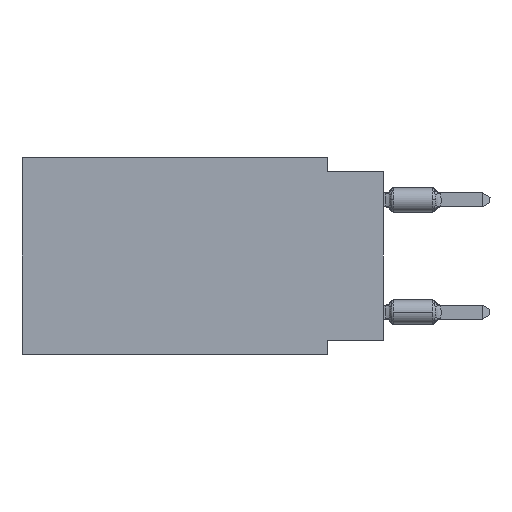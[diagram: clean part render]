
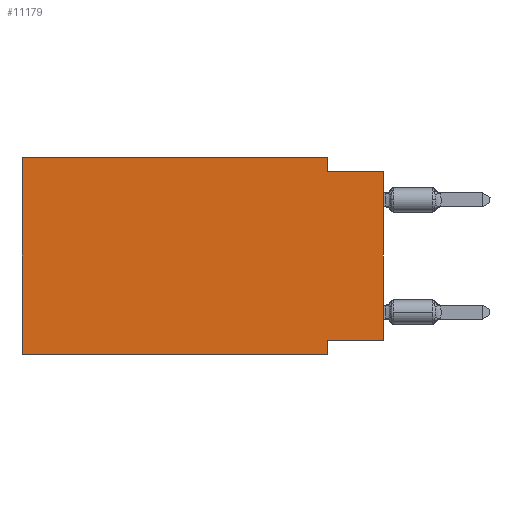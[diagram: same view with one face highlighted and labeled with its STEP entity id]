
A CAD part, left-side view. The second image highlights one B-rep face of the part: STEP entity #11179.
In plain terms, the highlighted planar face has unit normal (-1, 0, 0).
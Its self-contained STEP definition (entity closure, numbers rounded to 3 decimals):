
#908 = DIRECTION ( 'NONE',  ( 0., 0., -1. ) ) ;
#1858 = LINE ( 'NONE', #10172, #21087 ) ;
#2636 = DIRECTION ( 'NONE',  ( 0., 1., 0. ) ) ;
#2695 = VERTEX_POINT ( 'NONE', #25205 ) ;
#3220 = LINE ( 'NONE', #24862, #30269 ) ;
#4189 = VECTOR ( 'NONE', #20116, 1000. ) ;
#4745 = VERTEX_POINT ( 'NONE', #19446 ) ;
#5129 = LINE ( 'NONE', #21970, #16484 ) ;
#6118 = CARTESIAN_POINT ( 'NONE',  ( 0., 0., -0.635 ) ) ;
#7174 = DIRECTION ( 'NONE',  ( 0., 0., -1. ) ) ;
#7586 = ORIENTED_EDGE ( 'NONE', *, *, #32528, .F. ) ;
#7727 = CARTESIAN_POINT ( 'NONE',  ( 0., 2.54, -8.255 ) ) ;
#9203 = EDGE_CURVE ( 'NONE', #30146, #4745, #13804, .T. ) ;
#9887 = DIRECTION ( 'NONE',  ( 0., 0., -1. ) ) ;
#10009 = DIRECTION ( 'NONE',  ( 0., -1., 0. ) ) ;
#10089 = CARTESIAN_POINT ( 'NONE',  ( 0., 0., -8.255 ) ) ;
#10172 = CARTESIAN_POINT ( 'NONE',  ( 0., 16.383, 0. ) ) ;
#10361 = CARTESIAN_POINT ( 'NONE',  ( 0., 16.383, -8.89 ) ) ;
#11179 = ADVANCED_FACE ( 'NONE', ( #23169 ), #29033, .F. ) ;
#12017 = ORIENTED_EDGE ( 'NONE', *, *, #25292, .F. ) ;
#12849 = CARTESIAN_POINT ( 'NONE',  ( 0., 16.383, 0. ) ) ;
#13617 = ORIENTED_EDGE ( 'NONE', *, *, #9203, .T. ) ;
#13804 = LINE ( 'NONE', #29809, #14140 ) ;
#14010 = EDGE_CURVE ( 'NONE', #21302, #32073, #32221, .T. ) ;
#14140 = VECTOR ( 'NONE', #21966, 1000. ) ;
#16460 = VERTEX_POINT ( 'NONE', #17766 ) ;
#16484 = VECTOR ( 'NONE', #2636, 1000. ) ;
#16853 = EDGE_CURVE ( 'NONE', #17032, #32073, #20550, .T. ) ;
#16901 = CARTESIAN_POINT ( 'NONE',  ( 0., 16.383, 0. ) ) ;
#17032 = VERTEX_POINT ( 'NONE', #7727 ) ;
#17487 = LINE ( 'NONE', #6118, #27730 ) ;
#17766 = CARTESIAN_POINT ( 'NONE',  ( 0., 2.54, 0. ) ) ;
#19446 = CARTESIAN_POINT ( 'NONE',  ( 0., 0., -0.635 ) ) ;
#19974 = ORIENTED_EDGE ( 'NONE', *, *, #16853, .F. ) ;
#20116 = DIRECTION ( 'NONE',  ( 0., -1., 0. ) ) ;
#20370 = CARTESIAN_POINT ( 'NONE',  ( 0., 2.54, -8.89 ) ) ;
#20550 = LINE ( 'NONE', #31224, #26715 ) ;
#21087 = VECTOR ( 'NONE', #28681, 1000. ) ;
#21229 = ORIENTED_EDGE ( 'NONE', *, *, #22100, .F. ) ;
#21302 = VERTEX_POINT ( 'NONE', #29407 ) ;
#21428 = ORIENTED_EDGE ( 'NONE', *, *, #29186, .F. ) ;
#21966 = DIRECTION ( 'NONE',  ( 0., 0., 1. ) ) ;
#21970 = CARTESIAN_POINT ( 'NONE',  ( 0., 0., -8.255 ) ) ;
#22100 = EDGE_CURVE ( 'NONE', #30146, #17032, #5129, .T. ) ;
#23169 = FACE_OUTER_BOUND ( 'NONE', #23328, .T. ) ;
#23328 = EDGE_LOOP ( 'NONE', ( #13617, #7586, #12017, #30321, #21428, #34111, #19974, #21229 ) ) ;
#24862 = CARTESIAN_POINT ( 'NONE',  ( 0., 2.54, 0. ) ) ;
#24988 = EDGE_CURVE ( 'NONE', #31687, #16460, #34009, .T. ) ;
#25205 = CARTESIAN_POINT ( 'NONE',  ( 0., 2.54, -0.635 ) ) ;
#25292 = EDGE_CURVE ( 'NONE', #16460, #2695, #3220, .T. ) ;
#25366 = VECTOR ( 'NONE', #10009, 1000. ) ;
#26715 = VECTOR ( 'NONE', #9887, 1000. ) ;
#27730 = VECTOR ( 'NONE', #27982, 1000. ) ;
#27982 = DIRECTION ( 'NONE',  ( 0., -1., 0. ) ) ;
#28133 = AXIS2_PLACEMENT_3D ( 'NONE', #12849, #28684, #7174 ) ;
#28655 = CARTESIAN_POINT ( 'NONE',  ( 0., 16.383, 0. ) ) ;
#28681 = DIRECTION ( 'NONE',  ( 0., 0., 1. ) ) ;
#28684 = DIRECTION ( 'NONE',  ( 1., 0., 0. ) ) ;
#29033 = PLANE ( 'NONE',  #28133 ) ;
#29186 = EDGE_CURVE ( 'NONE', #21302, #31687, #1858, .T. ) ;
#29407 = CARTESIAN_POINT ( 'NONE',  ( 0., 16.383, -8.89 ) ) ;
#29809 = CARTESIAN_POINT ( 'NONE',  ( 0., 0., 0. ) ) ;
#30146 = VERTEX_POINT ( 'NONE', #10089 ) ;
#30269 = VECTOR ( 'NONE', #908, 1000. ) ;
#30321 = ORIENTED_EDGE ( 'NONE', *, *, #24988, .F. ) ;
#31224 = CARTESIAN_POINT ( 'NONE',  ( 0., 2.54, -8.89 ) ) ;
#31687 = VERTEX_POINT ( 'NONE', #16901 ) ;
#32073 = VERTEX_POINT ( 'NONE', #20370 ) ;
#32221 = LINE ( 'NONE', #10361, #25366 ) ;
#32528 = EDGE_CURVE ( 'NONE', #2695, #4745, #17487, .T. ) ;
#34009 = LINE ( 'NONE', #28655, #4189 ) ;
#34111 = ORIENTED_EDGE ( 'NONE', *, *, #14010, .T. ) ;
